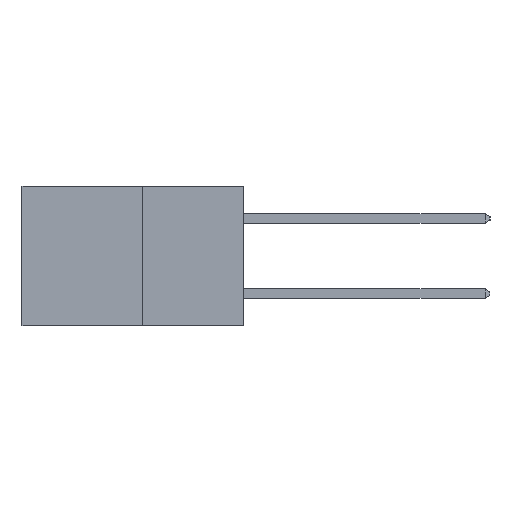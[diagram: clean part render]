
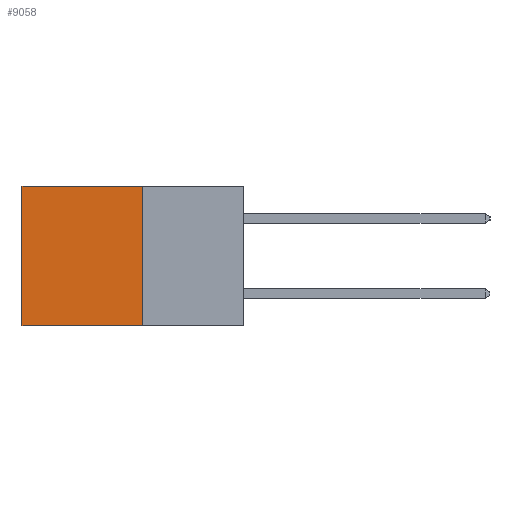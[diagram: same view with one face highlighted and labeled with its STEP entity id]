
A CAD part, left-side view. The second image highlights one B-rep face of the part: STEP entity #9058.
In plain terms, the highlighted planar face has unit normal (-1, 0, 0).
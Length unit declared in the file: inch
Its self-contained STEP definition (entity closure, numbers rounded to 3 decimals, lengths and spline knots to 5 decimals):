
#148 = FACE_OUTER_BOUND ( 'NONE', #1454, .T. ) ;
#473 = CARTESIAN_POINT ( 'NONE',  ( 0.277, 0.27, 0. ) ) ;
#913 = LINE ( 'NONE', #5802, #5280 ) ;
#1454 = EDGE_LOOP ( 'NONE', ( #6013, #5913, #5901, #10415 ) ) ;
#2535 = EDGE_CURVE ( 'NONE', #9508, #3440, #7998, .T. ) ;
#2937 = LINE ( 'NONE', #7162, #5345 ) ;
#3054 = EDGE_CURVE ( 'NONE', #9508, #3850, #913, .T. ) ;
#3378 = VECTOR ( 'NONE', #9207, 39.37008 ) ;
#3440 = VERTEX_POINT ( 'NONE', #4674 ) ;
#3850 = VERTEX_POINT ( 'NONE', #7697 ) ;
#3962 = LINE ( 'NONE', #7254, #6215 ) ;
#4674 = CARTESIAN_POINT ( 'NONE',  ( 0.277, 0.27, -0.37 ) ) ;
#5280 = VECTOR ( 'NONE', #5754, 39.37008 ) ;
#5345 = VECTOR ( 'NONE', #7155, 39.37008 ) ;
#5451 = AXIS2_PLACEMENT_3D ( 'NONE', #7253, #6583, #6350 ) ;
#5754 = DIRECTION ( 'NONE',  ( 0., 1., 0. ) ) ;
#5802 = CARTESIAN_POINT ( 'NONE',  ( 0.277, 0.27, 0. ) ) ;
#5901 = ORIENTED_EDGE ( 'NONE', *, *, #2535, .F. ) ;
#5913 = ORIENTED_EDGE ( 'NONE', *, *, #6283, .F. ) ;
#6013 = ORIENTED_EDGE ( 'NONE', *, *, #8788, .T. ) ;
#6215 = VECTOR ( 'NONE', #7791, 39.37008 ) ;
#6283 = EDGE_CURVE ( 'NONE', #3440, #7970, #2937, .T. ) ;
#6350 = DIRECTION ( 'NONE',  ( 0., 0., -1. ) ) ;
#6583 = DIRECTION ( 'NONE',  ( 1., 0., 0. ) ) ;
#6864 = PLANE ( 'NONE',  #5451 ) ;
#7155 = DIRECTION ( 'NONE',  ( 0., 1., 0. ) ) ;
#7162 = CARTESIAN_POINT ( 'NONE',  ( 0.277, 0.27, -0.37 ) ) ;
#7253 = CARTESIAN_POINT ( 'NONE',  ( 0.277, 0.27, -0.37 ) ) ;
#7254 = CARTESIAN_POINT ( 'NONE',  ( 0.277, 0.59, -0.37 ) ) ;
#7697 = CARTESIAN_POINT ( 'NONE',  ( 0.277, 0.59, 0. ) ) ;
#7791 = DIRECTION ( 'NONE',  ( 0., 0., -1. ) ) ;
#7970 = VERTEX_POINT ( 'NONE', #9781 ) ;
#7998 = LINE ( 'NONE', #10202, #3378 ) ;
#8788 = EDGE_CURVE ( 'NONE', #3850, #7970, #3962, .T. ) ;
#9058 = ADVANCED_FACE ( 'NONE', ( #148 ), #6864, .F. ) ;
#9207 = DIRECTION ( 'NONE',  ( 0., 0., -1. ) ) ;
#9508 = VERTEX_POINT ( 'NONE', #473 ) ;
#9781 = CARTESIAN_POINT ( 'NONE',  ( 0.277, 0.59, -0.37 ) ) ;
#10202 = CARTESIAN_POINT ( 'NONE',  ( 0.277, 0.27, -0.37 ) ) ;
#10415 = ORIENTED_EDGE ( 'NONE', *, *, #3054, .T. ) ;
